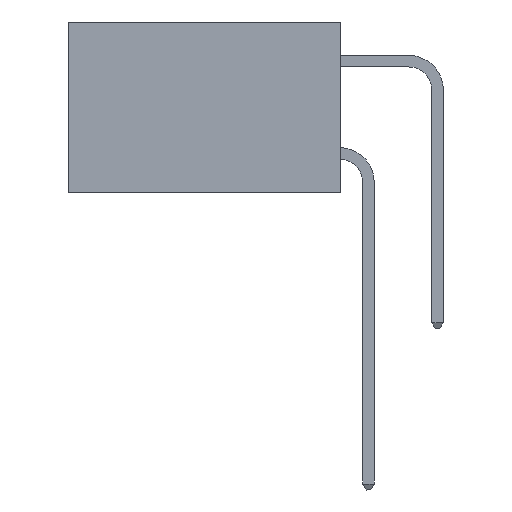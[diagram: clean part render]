
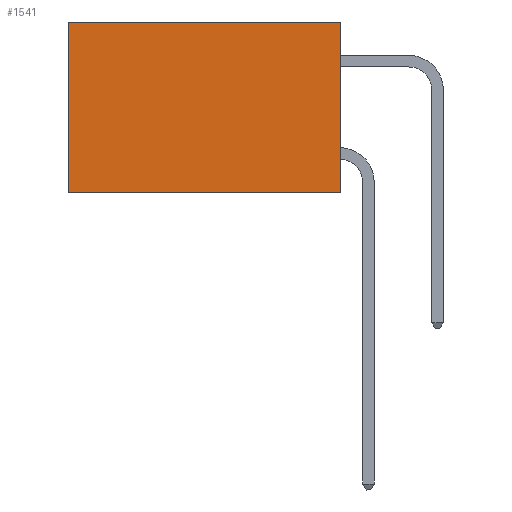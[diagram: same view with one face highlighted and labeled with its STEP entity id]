
A CAD part, left-side view. The second image highlights one B-rep face of the part: STEP entity #1541.
In plain terms, the highlighted planar face has unit normal (-1, 0, 0).
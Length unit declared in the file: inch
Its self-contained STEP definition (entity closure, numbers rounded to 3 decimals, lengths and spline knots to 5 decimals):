
#287 = ORIENTED_EDGE ( 'NONE', *, *, #9985, .F. ) ;
#378 = DIRECTION ( 'NONE',  ( 0., 1., 0. ) ) ;
#401 = EDGE_LOOP ( 'NONE', ( #2493, #3634, #287, #1388 ) ) ;
#855 = CARTESIAN_POINT ( 'NONE',  ( 0.277, 0.59, -0.37 ) ) ;
#1255 = EDGE_CURVE ( 'NONE', #7592, #12619, #7230, .T. ) ;
#1388 = ORIENTED_EDGE ( 'NONE', *, *, #8841, .T. ) ;
#1541 = ADVANCED_FACE ( 'NONE', ( #9451 ), #15020, .F. ) ;
#2493 = ORIENTED_EDGE ( 'NONE', *, *, #1255, .T. ) ;
#2687 = CARTESIAN_POINT ( 'NONE',  ( 0.277, 0., -0.37 ) ) ;
#3059 = CARTESIAN_POINT ( 'NONE',  ( 0.277, 0., 0. ) ) ;
#3437 = VECTOR ( 'NONE', #6240, 39.37008 ) ;
#3634 = ORIENTED_EDGE ( 'NONE', *, *, #9011, .F. ) ;
#4660 = CARTESIAN_POINT ( 'NONE',  ( 0.277, 0.59, -0.37 ) ) ;
#4715 = DIRECTION ( 'NONE',  ( 0., 0., -1. ) ) ;
#5966 = CARTESIAN_POINT ( 'NONE',  ( 0.277, 0., 0. ) ) ;
#6240 = DIRECTION ( 'NONE',  ( 0., 0., -1. ) ) ;
#6594 = VERTEX_POINT ( 'NONE', #3059 ) ;
#7230 = LINE ( 'NONE', #4660, #10033 ) ;
#7592 = VERTEX_POINT ( 'NONE', #8221 ) ;
#8221 = CARTESIAN_POINT ( 'NONE',  ( 0.277, 0.59, 0. ) ) ;
#8841 = EDGE_CURVE ( 'NONE', #6594, #7592, #9160, .T. ) ;
#9011 = EDGE_CURVE ( 'NONE', #13637, #12619, #12734, .T. ) ;
#9160 = LINE ( 'NONE', #5966, #12247 ) ;
#9451 = FACE_OUTER_BOUND ( 'NONE', #401, .T. ) ;
#9725 = VECTOR ( 'NONE', #378, 39.37008 ) ;
#9985 = EDGE_CURVE ( 'NONE', #6594, #13637, #12710, .T. ) ;
#10033 = VECTOR ( 'NONE', #4715, 39.37008 ) ;
#10343 = AXIS2_PLACEMENT_3D ( 'NONE', #14874, #14014, #13967 ) ;
#10946 = CARTESIAN_POINT ( 'NONE',  ( 0.277, 0., -0.37 ) ) ;
#12247 = VECTOR ( 'NONE', #14013, 39.37008 ) ;
#12619 = VERTEX_POINT ( 'NONE', #855 ) ;
#12710 = LINE ( 'NONE', #2687, #3437 ) ;
#12734 = LINE ( 'NONE', #14263, #9725 ) ;
#13637 = VERTEX_POINT ( 'NONE', #10946 ) ;
#13967 = DIRECTION ( 'NONE',  ( 0., 0., -1. ) ) ;
#14013 = DIRECTION ( 'NONE',  ( 0., 1., 0. ) ) ;
#14014 = DIRECTION ( 'NONE',  ( 1., 0., 0. ) ) ;
#14263 = CARTESIAN_POINT ( 'NONE',  ( 0.277, 0., -0.37 ) ) ;
#14874 = CARTESIAN_POINT ( 'NONE',  ( 0.277, 0., -0.37 ) ) ;
#15020 = PLANE ( 'NONE',  #10343 ) ;
